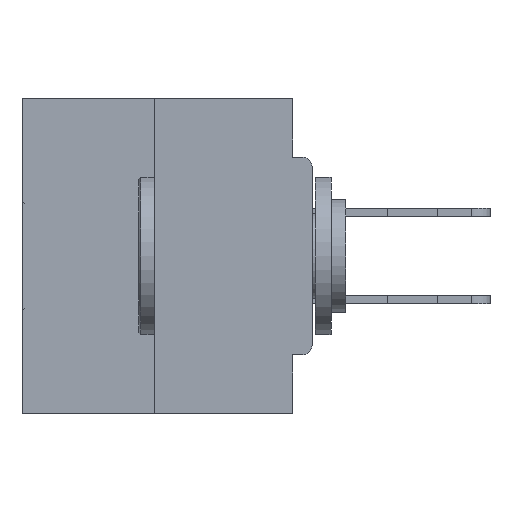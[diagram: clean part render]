
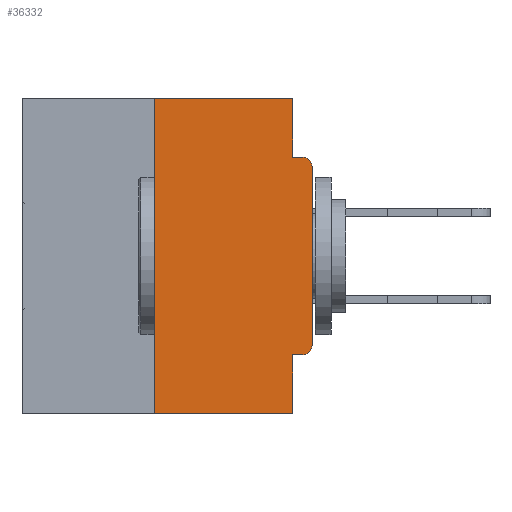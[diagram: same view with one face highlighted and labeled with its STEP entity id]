
A CAD part, left-side view. The second image highlights one B-rep face of the part: STEP entity #36332.
In plain terms, the highlighted planar face has unit normal (-1, 0, 0).
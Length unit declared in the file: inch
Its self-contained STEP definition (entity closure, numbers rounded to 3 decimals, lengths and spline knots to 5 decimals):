
#124 = VERTEX_POINT ( 'NONE', #10019 ) ;
#877 = DIRECTION ( 'NONE',  ( 0., 1., 0. ) ) ;
#1525 = AXIS2_PLACEMENT_3D ( 'NONE', #37060, #39900, #20568 ) ;
#2168 = DIRECTION ( 'NONE',  ( 0., -1., 0. ) ) ;
#2333 = LINE ( 'NONE', #16468, #36121 ) ;
#2785 = CARTESIAN_POINT ( 'NONE',  ( 0., 0., 0. ) ) ;
#2816 = CARTESIAN_POINT ( 'NONE',  ( 0., 0.015, -0.4065 ) ) ;
#3090 = EDGE_CURVE ( 'NONE', #16720, #6358, #31081, .T. ) ;
#3227 = PLANE ( 'NONE',  #24592 ) ;
#4691 = EDGE_CURVE ( 'NONE', #20353, #22221, #13262, .T. ) ;
#5132 = CARTESIAN_POINT ( 'NONE',  ( 0., 0.46, 0. ) ) ;
#6057 = LINE ( 'NONE', #15553, #19179 ) ;
#6358 = VERTEX_POINT ( 'NONE', #19186 ) ;
#7676 = LINE ( 'NONE', #26767, #15229 ) ;
#8376 = VECTOR ( 'NONE', #30499, 39.37008 ) ;
#8432 = ORIENTED_EDGE ( 'NONE', *, *, #38263, .T. ) ;
#9085 = VERTEX_POINT ( 'NONE', #35115 ) ;
#9169 = DIRECTION ( 'NONE',  ( 0., 0., -1. ) ) ;
#9479 = VECTOR ( 'NONE', #25329, 39.37008 ) ;
#9673 = DIRECTION ( 'NONE',  ( 0., 0., -1. ) ) ;
#10019 = CARTESIAN_POINT ( 'NONE',  ( 0., 0., -0.3915 ) ) ;
#10852 = CARTESIAN_POINT ( 'NONE',  ( 0., 0., -0.1085 ) ) ;
#11209 = CIRCLE ( 'NONE', #29200, 0.015 ) ;
#12013 = EDGE_CURVE ( 'NONE', #16720, #20392, #7676, .T. ) ;
#12476 = FACE_OUTER_BOUND ( 'NONE', #39339, .T. ) ;
#12631 = VERTEX_POINT ( 'NONE', #2816 ) ;
#13262 = CIRCLE ( 'NONE', #1525, 0.015 ) ;
#14041 = DIRECTION ( 'NONE',  ( 0., 0., 1. ) ) ;
#15229 = VECTOR ( 'NONE', #14041, 39.37008 ) ;
#15553 = CARTESIAN_POINT ( 'NONE',  ( 0., 0.031, 0. ) ) ;
#15918 = DIRECTION ( 'NONE',  ( -1., 0., 0. ) ) ;
#16238 = EDGE_CURVE ( 'NONE', #20392, #17082, #24058, .T. ) ;
#16468 = CARTESIAN_POINT ( 'NONE',  ( 0., 0., -0.4065 ) ) ;
#16479 = CARTESIAN_POINT ( 'NONE',  ( 0., 0.46, -0.5 ) ) ;
#16720 = VERTEX_POINT ( 'NONE', #24101 ) ;
#17082 = VERTEX_POINT ( 'NONE', #38297 ) ;
#17111 = CARTESIAN_POINT ( 'NONE',  ( 0., 0.031, -0.5 ) ) ;
#17299 = VERTEX_POINT ( 'NONE', #37278 ) ;
#18362 = ORIENTED_EDGE ( 'NONE', *, *, #25493, .T. ) ;
#18517 = VECTOR ( 'NONE', #36190, 39.37008 ) ;
#19179 = VECTOR ( 'NONE', #38172, 39.37008 ) ;
#19186 = CARTESIAN_POINT ( 'NONE',  ( 0., 0.031, -0.5 ) ) ;
#19424 = DIRECTION ( 'NONE',  ( 1., 0., 0. ) ) ;
#20353 = VERTEX_POINT ( 'NONE', #10852 ) ;
#20392 = VERTEX_POINT ( 'NONE', #40823 ) ;
#20568 = DIRECTION ( 'NONE',  ( 0., 0., -1. ) ) ;
#21025 = ORIENTED_EDGE ( 'NONE', *, *, #4691, .T. ) ;
#22221 = VERTEX_POINT ( 'NONE', #29051 ) ;
#24058 = LINE ( 'NONE', #5132, #8376 ) ;
#24101 = CARTESIAN_POINT ( 'NONE',  ( 0., 0.25, -0.5 ) ) ;
#24592 = AXIS2_PLACEMENT_3D ( 'NONE', #29005, #19424, #9673 ) ;
#25329 = DIRECTION ( 'NONE',  ( 0., 0., 1. ) ) ;
#25404 = ORIENTED_EDGE ( 'NONE', *, *, #32071, .F. ) ;
#25493 = EDGE_CURVE ( 'NONE', #124, #20353, #35272, .T. ) ;
#26123 = DIRECTION ( 'NONE',  ( 0., -1., 0. ) ) ;
#26395 = VECTOR ( 'NONE', #2168, 39.37008 ) ;
#26767 = CARTESIAN_POINT ( 'NONE',  ( 0., 0.25, 0. ) ) ;
#27833 = CARTESIAN_POINT ( 'NONE',  ( 0., 0., -0.0935 ) ) ;
#27894 = ORIENTED_EDGE ( 'NONE', *, *, #29632, .F. ) ;
#29005 = CARTESIAN_POINT ( 'NONE',  ( 0., 0.46, 0. ) ) ;
#29051 = CARTESIAN_POINT ( 'NONE',  ( 0., 0.015, -0.0935 ) ) ;
#29200 = AXIS2_PLACEMENT_3D ( 'NONE', #38275, #15918, #9169 ) ;
#29575 = VECTOR ( 'NONE', #26123, 39.37008 ) ;
#29632 = EDGE_CURVE ( 'NONE', #9085, #6358, #33180, .T. ) ;
#30232 = ORIENTED_EDGE ( 'NONE', *, *, #3090, .T. ) ;
#30499 = DIRECTION ( 'NONE',  ( 0., -1., 0. ) ) ;
#30672 = EDGE_CURVE ( 'NONE', #12631, #9085, #2333, .T. ) ;
#31081 = LINE ( 'NONE', #16479, #29575 ) ;
#32071 = EDGE_CURVE ( 'NONE', #17299, #22221, #33456, .T. ) ;
#33180 = LINE ( 'NONE', #17111, #18517 ) ;
#33456 = LINE ( 'NONE', #27833, #26395 ) ;
#35115 = CARTESIAN_POINT ( 'NONE',  ( 0., 0.031, -0.4065 ) ) ;
#35272 = LINE ( 'NONE', #2785, #9479 ) ;
#35320 = ORIENTED_EDGE ( 'NONE', *, *, #39594, .F. ) ;
#36121 = VECTOR ( 'NONE', #877, 39.37008 ) ;
#36190 = DIRECTION ( 'NONE',  ( 0., 0., -1. ) ) ;
#36332 = ADVANCED_FACE ( 'NONE', ( #12476 ), #3227, .F. ) ;
#37060 = CARTESIAN_POINT ( 'NONE',  ( 0., 0.015, -0.1085 ) ) ;
#37218 = ORIENTED_EDGE ( 'NONE', *, *, #12013, .F. ) ;
#37278 = CARTESIAN_POINT ( 'NONE',  ( 0., 0.031, -0.0935 ) ) ;
#37429 = ORIENTED_EDGE ( 'NONE', *, *, #30672, .F. ) ;
#38172 = DIRECTION ( 'NONE',  ( 0., 0., -1. ) ) ;
#38263 = EDGE_CURVE ( 'NONE', #12631, #124, #11209, .T. ) ;
#38275 = CARTESIAN_POINT ( 'NONE',  ( 0., 0.015, -0.3915 ) ) ;
#38297 = CARTESIAN_POINT ( 'NONE',  ( 0., 0.031, 0. ) ) ;
#38304 = ORIENTED_EDGE ( 'NONE', *, *, #16238, .F. ) ;
#39339 = EDGE_LOOP ( 'NONE', ( #38304, #37218, #30232, #27894, #37429, #8432, #18362, #21025, #25404, #35320 ) ) ;
#39594 = EDGE_CURVE ( 'NONE', #17082, #17299, #6057, .T. ) ;
#39900 = DIRECTION ( 'NONE',  ( -1., 0., 0. ) ) ;
#40823 = CARTESIAN_POINT ( 'NONE',  ( 0., 0.25, 0. ) ) ;
